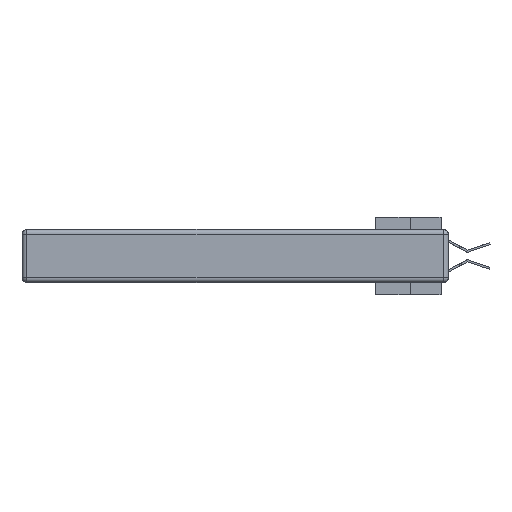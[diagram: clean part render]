
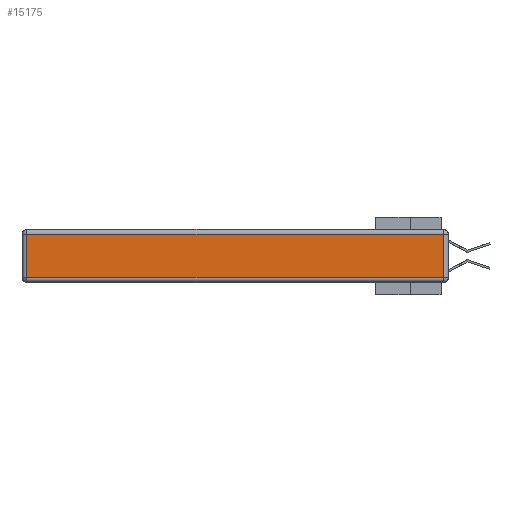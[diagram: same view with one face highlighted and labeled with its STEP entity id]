
A CAD part, left-side view. The second image highlights one B-rep face of the part: STEP entity #15175.
In plain terms, the highlighted planar face has unit normal (-1, 0, 0).
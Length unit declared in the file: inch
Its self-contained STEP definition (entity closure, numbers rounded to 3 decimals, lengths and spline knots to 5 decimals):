
#1433 = LINE ( 'NONE', #10226, #33589 ) ;
#1687 = VERTEX_POINT ( 'NONE', #5478 ) ;
#2360 = CARTESIAN_POINT ( 'NONE',  ( 0., 0., -0.313 ) ) ;
#3973 = EDGE_CURVE ( 'NONE', #1687, #20574, #35006, .T. ) ;
#4892 = EDGE_CURVE ( 'NONE', #20574, #33246, #1433, .T. ) ;
#4951 = CARTESIAN_POINT ( 'NONE',  ( 0., 2.72, -0.313 ) ) ;
#5478 = CARTESIAN_POINT ( 'NONE',  ( 0., 0.03, -0.313 ) ) ;
#6482 = CARTESIAN_POINT ( 'NONE',  ( 0., 0.03, -0.343 ) ) ;
#7546 = DIRECTION ( 'NONE',  ( -1., 0., 0. ) ) ;
#8429 = CARTESIAN_POINT ( 'NONE',  ( 0., 2.72, -0.03 ) ) ;
#9969 = VECTOR ( 'NONE', #11392, 39.37008 ) ;
#10226 = CARTESIAN_POINT ( 'NONE',  ( 0., 2.75, -0.03 ) ) ;
#10434 = CARTESIAN_POINT ( 'NONE',  ( 0., 0.03, -0.03 ) ) ;
#11021 = EDGE_CURVE ( 'NONE', #33246, #21018, #19601, .T. ) ;
#11037 = CARTESIAN_POINT ( 'NONE',  ( 0., 2.72, -0.343 ) ) ;
#11392 = DIRECTION ( 'NONE',  ( 0., 0., -1. ) ) ;
#13912 = DIRECTION ( 'NONE',  ( 0., 0., 1. ) ) ;
#13965 = ORIENTED_EDGE ( 'NONE', *, *, #22389, .T. ) ;
#15021 = EDGE_LOOP ( 'NONE', ( #13965, #24296, #35443, #25155 ) ) ;
#15175 = ADVANCED_FACE ( 'NONE', ( #21908 ), #36432, .T. ) ;
#19601 = LINE ( 'NONE', #11037, #9969 ) ;
#20574 = VERTEX_POINT ( 'NONE', #10434 ) ;
#21018 = VERTEX_POINT ( 'NONE', #4951 ) ;
#21020 = VECTOR ( 'NONE', #35951, 39.37008 ) ;
#21398 = AXIS2_PLACEMENT_3D ( 'NONE', #33083, #7546, #13912 ) ;
#21599 = DIRECTION ( 'NONE',  ( 0., 1., 0. ) ) ;
#21908 = FACE_OUTER_BOUND ( 'NONE', #15021, .T. ) ;
#22389 = EDGE_CURVE ( 'NONE', #21018, #1687, #25505, .T. ) ;
#23307 = VECTOR ( 'NONE', #29422, 39.37008 ) ;
#24296 = ORIENTED_EDGE ( 'NONE', *, *, #3973, .T. ) ;
#25155 = ORIENTED_EDGE ( 'NONE', *, *, #11021, .T. ) ;
#25505 = LINE ( 'NONE', #2360, #21020 ) ;
#29422 = DIRECTION ( 'NONE',  ( 0., 0., 1. ) ) ;
#33083 = CARTESIAN_POINT ( 'NONE',  ( 0., 0., -0.343 ) ) ;
#33246 = VERTEX_POINT ( 'NONE', #8429 ) ;
#33589 = VECTOR ( 'NONE', #21599, 39.37008 ) ;
#35006 = LINE ( 'NONE', #6482, #23307 ) ;
#35443 = ORIENTED_EDGE ( 'NONE', *, *, #4892, .T. ) ;
#35951 = DIRECTION ( 'NONE',  ( 0., -1., 0. ) ) ;
#36432 = PLANE ( 'NONE',  #21398 ) ;
